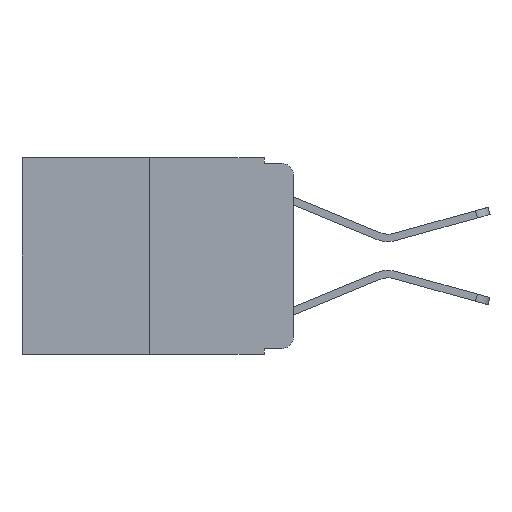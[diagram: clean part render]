
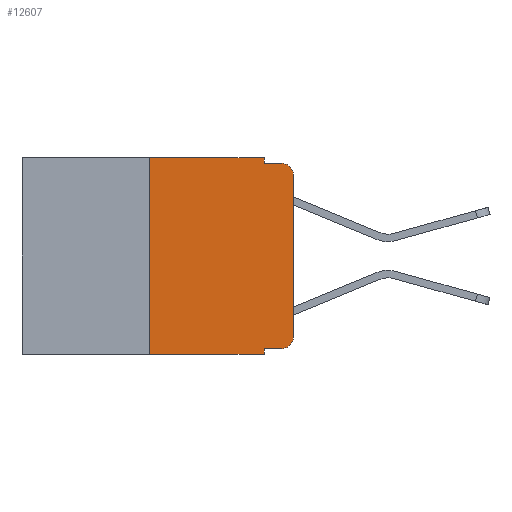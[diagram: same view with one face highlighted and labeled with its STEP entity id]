
A CAD part, left-side view. The second image highlights one B-rep face of the part: STEP entity #12607.
In plain terms, the highlighted planar face has unit normal (-1, 0, 0).
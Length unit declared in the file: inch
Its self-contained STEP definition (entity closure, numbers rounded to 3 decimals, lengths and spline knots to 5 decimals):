
#57 = EDGE_CURVE ( 'NONE', #6747, #1888, #6421, .T. ) ;
#114 = AXIS2_PLACEMENT_3D ( 'NONE', #6903, #6129, #6970 ) ;
#243 = CARTESIAN_POINT ( 'NONE',  ( 0., 0.051, 0. ) ) ;
#297 = ORIENTED_EDGE ( 'NONE', *, *, #1590, .T. ) ;
#303 = DIRECTION ( 'NONE',  ( 0., -1., 0. ) ) ;
#557 = VECTOR ( 'NONE', #6518, 39.37008 ) ;
#904 = DIRECTION ( 'NONE',  ( 1., 0., 0. ) ) ;
#1069 = AXIS2_PLACEMENT_3D ( 'NONE', #7869, #904, #4670 ) ;
#1079 = CARTESIAN_POINT ( 'NONE',  ( 0., 0.051, -0.01 ) ) ;
#1436 = ORIENTED_EDGE ( 'NONE', *, *, #5366, .F. ) ;
#1590 = EDGE_CURVE ( 'NONE', #6747, #4658, #8837, .T. ) ;
#1888 = VERTEX_POINT ( 'NONE', #13085 ) ;
#2022 = DIRECTION ( 'NONE',  ( 0., 0., -1. ) ) ;
#2112 = ORIENTED_EDGE ( 'NONE', *, *, #2947, .T. ) ;
#2166 = FACE_OUTER_BOUND ( 'NONE', #9141, .T. ) ;
#2211 = CARTESIAN_POINT ( 'NONE',  ( 0., 0.473, -0.343 ) ) ;
#2810 = CARTESIAN_POINT ( 'NONE',  ( 0., 0.25, 0. ) ) ;
#2947 = EDGE_CURVE ( 'NONE', #8382, #3005, #4543, .T. ) ;
#3005 = VERTEX_POINT ( 'NONE', #7686 ) ;
#3070 = ORIENTED_EDGE ( 'NONE', *, *, #4906, .T. ) ;
#3108 = DIRECTION ( 'NONE',  ( 0., -1., 0. ) ) ;
#3169 = VERTEX_POINT ( 'NONE', #11570 ) ;
#3195 = CARTESIAN_POINT ( 'NONE',  ( 0., 0., 0. ) ) ;
#3381 = ORIENTED_EDGE ( 'NONE', *, *, #6689, .T. ) ;
#3476 = DIRECTION ( 'NONE',  ( 0., -1., 0. ) ) ;
#3620 = CARTESIAN_POINT ( 'NONE',  ( 0., 0.051, -0.333 ) ) ;
#3919 = ORIENTED_EDGE ( 'NONE', *, *, #4781, .F. ) ;
#4345 = VECTOR ( 'NONE', #6384, 39.37008 ) ;
#4364 = VECTOR ( 'NONE', #14670, 39.37008 ) ;
#4543 = LINE ( 'NONE', #3195, #6717 ) ;
#4658 = VERTEX_POINT ( 'NONE', #7546 ) ;
#4670 = DIRECTION ( 'NONE',  ( 0., 0., -1. ) ) ;
#4781 = EDGE_CURVE ( 'NONE', #10749, #14409, #10039, .T. ) ;
#4906 = EDGE_CURVE ( 'NONE', #3169, #5430, #12985, .T. ) ;
#5366 = EDGE_CURVE ( 'NONE', #3169, #4658, #9998, .T. ) ;
#5430 = VERTEX_POINT ( 'NONE', #10229 ) ;
#6129 = DIRECTION ( 'NONE',  ( -1., 0., 0. ) ) ;
#6384 = DIRECTION ( 'NONE',  ( 0., 0., -1. ) ) ;
#6421 = LINE ( 'NONE', #2810, #8881 ) ;
#6518 = DIRECTION ( 'NONE',  ( 0., 0., -1. ) ) ;
#6689 = EDGE_CURVE ( 'NONE', #5430, #8382, #8256, .T. ) ;
#6717 = VECTOR ( 'NONE', #14683, 39.37008 ) ;
#6747 = VERTEX_POINT ( 'NONE', #9320 ) ;
#6903 = CARTESIAN_POINT ( 'NONE',  ( 0., 0.02, -0.03 ) ) ;
#6970 = DIRECTION ( 'NONE',  ( 0., 0., -1. ) ) ;
#7075 = LINE ( 'NONE', #11831, #7099 ) ;
#7099 = VECTOR ( 'NONE', #303, 39.37008 ) ;
#7264 = ORIENTED_EDGE ( 'NONE', *, *, #11923, .T. ) ;
#7428 = VECTOR ( 'NONE', #3108, 39.37008 ) ;
#7546 = CARTESIAN_POINT ( 'NONE',  ( 0., 0.051, -0.343 ) ) ;
#7604 = CARTESIAN_POINT ( 'NONE',  ( 0., 0.051, -0.01 ) ) ;
#7686 = CARTESIAN_POINT ( 'NONE',  ( 0., 0., -0.03 ) ) ;
#7780 = CARTESIAN_POINT ( 'NONE',  ( 0., 0., -0.313 ) ) ;
#7806 = PLANE ( 'NONE',  #1069 ) ;
#7869 = CARTESIAN_POINT ( 'NONE',  ( 0., 0.473, 0. ) ) ;
#8256 = CIRCLE ( 'NONE', #11671, 0.02 ) ;
#8382 = VERTEX_POINT ( 'NONE', #7780 ) ;
#8580 = CARTESIAN_POINT ( 'NONE',  ( 0., 0.051, 0. ) ) ;
#8837 = LINE ( 'NONE', #2211, #7428 ) ;
#8881 = VECTOR ( 'NONE', #12017, 39.37008 ) ;
#8943 = CARTESIAN_POINT ( 'NONE',  ( 0., 0.02, -0.313 ) ) ;
#9141 = EDGE_LOOP ( 'NONE', ( #2112, #7264, #3919, #11492, #13338, #14662, #297, #1436, #3070, #3381 ) ) ;
#9320 = CARTESIAN_POINT ( 'NONE',  ( 0., 0.25, -0.343 ) ) ;
#9712 = LINE ( 'NONE', #243, #4345 ) ;
#9998 = LINE ( 'NONE', #12559, #557 ) ;
#10039 = LINE ( 'NONE', #1079, #4364 ) ;
#10229 = CARTESIAN_POINT ( 'NONE',  ( 0., 0.02, -0.333 ) ) ;
#10749 = VERTEX_POINT ( 'NONE', #7604 ) ;
#10841 = CARTESIAN_POINT ( 'NONE',  ( 0., 0.02, -0.01 ) ) ;
#11281 = VERTEX_POINT ( 'NONE', #8580 ) ;
#11492 = ORIENTED_EDGE ( 'NONE', *, *, #14426, .F. ) ;
#11570 = CARTESIAN_POINT ( 'NONE',  ( 0., 0.051, -0.333 ) ) ;
#11619 = VECTOR ( 'NONE', #3476, 39.37008 ) ;
#11671 = AXIS2_PLACEMENT_3D ( 'NONE', #8943, #12348, #2022 ) ;
#11831 = CARTESIAN_POINT ( 'NONE',  ( 0., 0.473, 0. ) ) ;
#11923 = EDGE_CURVE ( 'NONE', #3005, #14409, #14342, .T. ) ;
#12017 = DIRECTION ( 'NONE',  ( 0., 0., 1. ) ) ;
#12348 = DIRECTION ( 'NONE',  ( -1., 0., 0. ) ) ;
#12559 = CARTESIAN_POINT ( 'NONE',  ( 0., 0.051, 0. ) ) ;
#12607 = ADVANCED_FACE ( 'NONE', ( #2166 ), #7806, .F. ) ;
#12816 = EDGE_CURVE ( 'NONE', #1888, #11281, #7075, .T. ) ;
#12985 = LINE ( 'NONE', #3620, #11619 ) ;
#13085 = CARTESIAN_POINT ( 'NONE',  ( 0., 0.25, 0. ) ) ;
#13338 = ORIENTED_EDGE ( 'NONE', *, *, #12816, .F. ) ;
#14342 = CIRCLE ( 'NONE', #114, 0.02 ) ;
#14409 = VERTEX_POINT ( 'NONE', #10841 ) ;
#14426 = EDGE_CURVE ( 'NONE', #11281, #10749, #9712, .T. ) ;
#14662 = ORIENTED_EDGE ( 'NONE', *, *, #57, .F. ) ;
#14670 = DIRECTION ( 'NONE',  ( 0., -1., 0. ) ) ;
#14683 = DIRECTION ( 'NONE',  ( 0., 0., 1. ) ) ;
